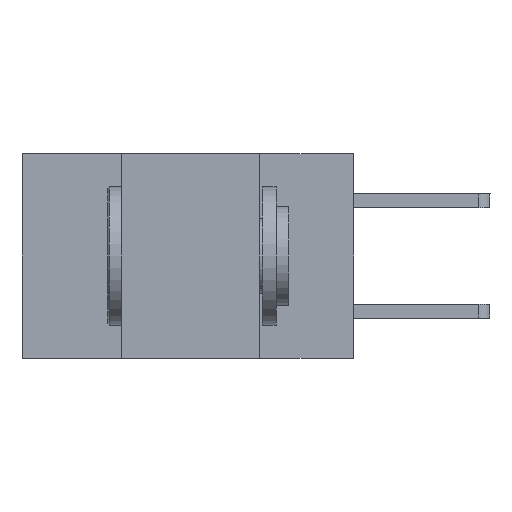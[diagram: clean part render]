
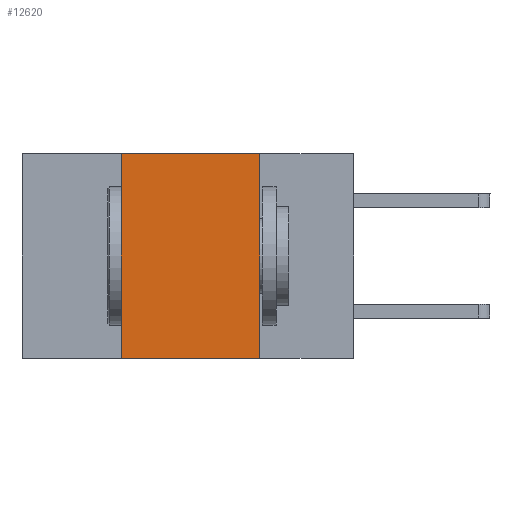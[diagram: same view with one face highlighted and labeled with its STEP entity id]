
A CAD part, left-side view. The second image highlights one B-rep face of the part: STEP entity #12620.
In plain terms, the highlighted planar face has unit normal (-1, 0, 0).
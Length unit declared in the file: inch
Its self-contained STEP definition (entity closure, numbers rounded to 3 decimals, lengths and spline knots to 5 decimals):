
#136 = ORIENTED_EDGE ( 'NONE', *, *, #14956, .F. ) ;
#842 = VECTOR ( 'NONE', #9739, 39.37008 ) ;
#1253 = CARTESIAN_POINT ( 'NONE',  ( 0., 0.17, 0. ) ) ;
#2780 = VERTEX_POINT ( 'NONE', #5567 ) ;
#2985 = CARTESIAN_POINT ( 'NONE',  ( 0., 0.17, -0.37 ) ) ;
#3014 = EDGE_LOOP ( 'NONE', ( #136, #12452, #11732, #5083 ) ) ;
#3029 = VECTOR ( 'NONE', #4319, 39.37008 ) ;
#3442 = CARTESIAN_POINT ( 'NONE',  ( 0., 0.42, 0. ) ) ;
#4200 = DIRECTION ( 'NONE',  ( 1., 0., 0. ) ) ;
#4319 = DIRECTION ( 'NONE',  ( 0., 0., 1. ) ) ;
#4606 = LINE ( 'NONE', #13737, #11245 ) ;
#4984 = VERTEX_POINT ( 'NONE', #2985 ) ;
#5045 = AXIS2_PLACEMENT_3D ( 'NONE', #7783, #4200, #12450 ) ;
#5070 = CARTESIAN_POINT ( 'NONE',  ( 0., 0.17, 0. ) ) ;
#5083 = ORIENTED_EDGE ( 'NONE', *, *, #12738, .T. ) ;
#5567 = CARTESIAN_POINT ( 'NONE',  ( 0., 0.42, -0.37 ) ) ;
#6389 = EDGE_CURVE ( 'NONE', #15485, #10050, #4606, .T. ) ;
#6808 = DIRECTION ( 'NONE',  ( 0., -1., 0. ) ) ;
#7697 = VECTOR ( 'NONE', #11473, 39.37008 ) ;
#7783 = CARTESIAN_POINT ( 'NONE',  ( 0., 0.6, 0. ) ) ;
#9075 = LINE ( 'NONE', #12561, #3029 ) ;
#9739 = DIRECTION ( 'NONE',  ( 0., 0., -1. ) ) ;
#10050 = VERTEX_POINT ( 'NONE', #5070 ) ;
#10291 = CARTESIAN_POINT ( 'NONE',  ( 0., 0.6, -0.37 ) ) ;
#10788 = LINE ( 'NONE', #10291, #7697 ) ;
#11245 = VECTOR ( 'NONE', #6808, 39.37008 ) ;
#11280 = PLANE ( 'NONE',  #5045 ) ;
#11473 = DIRECTION ( 'NONE',  ( 0., -1., 0. ) ) ;
#11732 = ORIENTED_EDGE ( 'NONE', *, *, #14223, .F. ) ;
#12450 = DIRECTION ( 'NONE',  ( 0., 0., -1. ) ) ;
#12452 = ORIENTED_EDGE ( 'NONE', *, *, #6389, .F. ) ;
#12561 = CARTESIAN_POINT ( 'NONE',  ( 0., 0.42, 0. ) ) ;
#12598 = FACE_OUTER_BOUND ( 'NONE', #3014, .T. ) ;
#12620 = ADVANCED_FACE ( 'NONE', ( #12598 ), #11280, .F. ) ;
#12738 = EDGE_CURVE ( 'NONE', #2780, #4984, #10788, .T. ) ;
#13270 = LINE ( 'NONE', #1253, #842 ) ;
#13737 = CARTESIAN_POINT ( 'NONE',  ( 0., 0.6, 0. ) ) ;
#14223 = EDGE_CURVE ( 'NONE', #2780, #15485, #9075, .T. ) ;
#14956 = EDGE_CURVE ( 'NONE', #10050, #4984, #13270, .T. ) ;
#15485 = VERTEX_POINT ( 'NONE', #3442 ) ;
